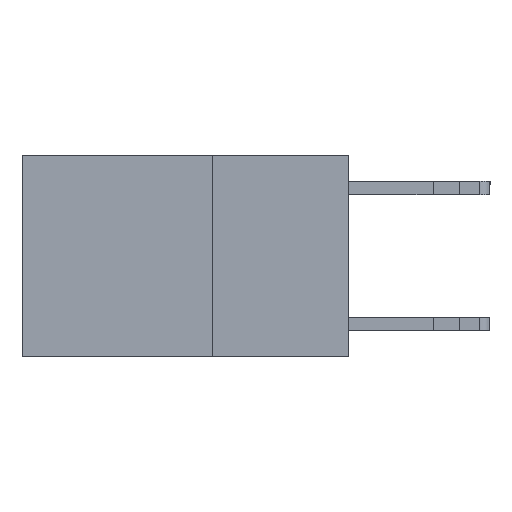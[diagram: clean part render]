
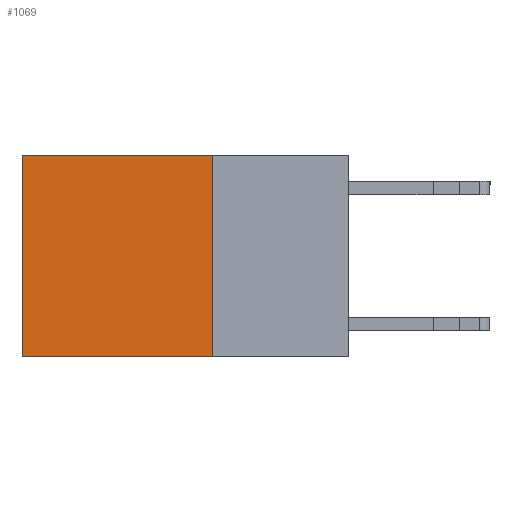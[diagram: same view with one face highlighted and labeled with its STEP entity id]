
A CAD part, left-side view. The second image highlights one B-rep face of the part: STEP entity #1069.
In plain terms, the highlighted planar face has unit normal (-1, 0, 0).
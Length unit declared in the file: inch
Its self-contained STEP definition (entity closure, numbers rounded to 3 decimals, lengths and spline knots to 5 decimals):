
#405 = DIRECTION ( 'NONE',  ( 0., 1., 0. ) ) ;
#1069 = ADVANCED_FACE ( 'NONE', ( #6156 ), #2990, .F. ) ;
#2890 = CARTESIAN_POINT ( 'NONE',  ( 0.2625, 0.25, 0. ) ) ;
#2905 = LINE ( 'NONE', #15332, #10911 ) ;
#2990 = PLANE ( 'NONE',  #7769 ) ;
#3362 = VECTOR ( 'NONE', #405, 39.37008 ) ;
#4157 = CARTESIAN_POINT ( 'NONE',  ( 0.2625, 0.25, 0. ) ) ;
#4372 = ORIENTED_EDGE ( 'NONE', *, *, #6246, .T. ) ;
#5565 = ORIENTED_EDGE ( 'NONE', *, *, #16843, .F. ) ;
#6130 = DIRECTION ( 'NONE',  ( 1., 0., 0. ) ) ;
#6156 = FACE_OUTER_BOUND ( 'NONE', #12885, .T. ) ;
#6206 = CARTESIAN_POINT ( 'NONE',  ( 0.2625, 0.25, 0. ) ) ;
#6233 = DIRECTION ( 'NONE',  ( 0., 0., -1. ) ) ;
#6246 = EDGE_CURVE ( 'NONE', #15060, #12607, #19395, .T. ) ;
#7769 = AXIS2_PLACEMENT_3D ( 'NONE', #10832, #6130, #6233 ) ;
#10360 = DIRECTION ( 'NONE',  ( 0., 0., -1. ) ) ;
#10507 = CARTESIAN_POINT ( 'NONE',  ( 0.2625, 0.6, -0.37 ) ) ;
#10832 = CARTESIAN_POINT ( 'NONE',  ( 0.2625, 0.25, 0. ) ) ;
#10911 = VECTOR ( 'NONE', #13295, 39.37008 ) ;
#11303 = LINE ( 'NONE', #15884, #3362 ) ;
#11448 = CARTESIAN_POINT ( 'NONE',  ( 0.2625, 0.25, -0.37 ) ) ;
#12563 = ORIENTED_EDGE ( 'NONE', *, *, #20067, .T. ) ;
#12607 = VERTEX_POINT ( 'NONE', #18575 ) ;
#12772 = VERTEX_POINT ( 'NONE', #11448 ) ;
#12885 = EDGE_LOOP ( 'NONE', ( #12563, #13020, #5565, #4372 ) ) ;
#13020 = ORIENTED_EDGE ( 'NONE', *, *, #15365, .F. ) ;
#13295 = DIRECTION ( 'NONE',  ( 0., 0., -1. ) ) ;
#13533 = LINE ( 'NONE', #4157, #18051 ) ;
#14569 = VERTEX_POINT ( 'NONE', #10507 ) ;
#15060 = VERTEX_POINT ( 'NONE', #6206 ) ;
#15332 = CARTESIAN_POINT ( 'NONE',  ( 0.2625, 0.6, 0. ) ) ;
#15365 = EDGE_CURVE ( 'NONE', #12772, #14569, #11303, .T. ) ;
#15884 = CARTESIAN_POINT ( 'NONE',  ( 0.2625, 0.25, -0.37 ) ) ;
#16843 = EDGE_CURVE ( 'NONE', #15060, #12772, #13533, .T. ) ;
#17874 = VECTOR ( 'NONE', #18275, 39.37008 ) ;
#18051 = VECTOR ( 'NONE', #10360, 39.37008 ) ;
#18275 = DIRECTION ( 'NONE',  ( 0., 1., 0. ) ) ;
#18575 = CARTESIAN_POINT ( 'NONE',  ( 0.2625, 0.6, 0. ) ) ;
#19395 = LINE ( 'NONE', #2890, #17874 ) ;
#20067 = EDGE_CURVE ( 'NONE', #12607, #14569, #2905, .T. ) ;
